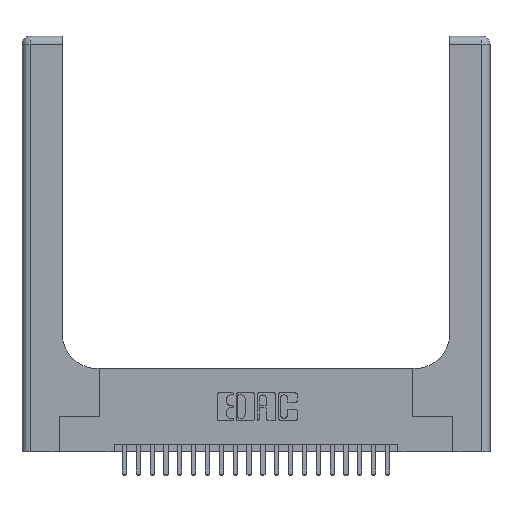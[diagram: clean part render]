
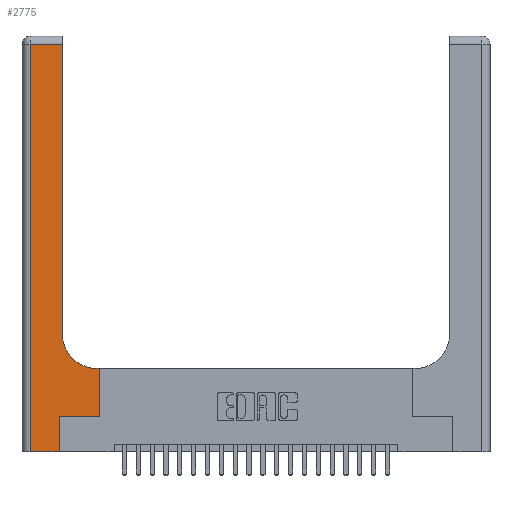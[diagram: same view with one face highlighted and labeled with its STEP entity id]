
A CAD part, top view. The second image highlights one B-rep face of the part: STEP entity #2775.
In plain terms, the highlighted planar face has unit normal (0, 0, 1).
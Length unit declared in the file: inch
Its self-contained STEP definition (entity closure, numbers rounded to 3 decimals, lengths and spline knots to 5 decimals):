
#641 = FACE_OUTER_BOUND ( 'NONE', #3121, .T. ) ;
#730 = VERTEX_POINT ( 'NONE', #21293 ) ;
#786 = ORIENTED_EDGE ( 'NONE', *, *, #1810, .T. ) ;
#1066 = CARTESIAN_POINT ( 'NONE',  ( 0., 3., 0.37 ) ) ;
#1249 = ORIENTED_EDGE ( 'NONE', *, *, #1352, .T. ) ;
#1352 = EDGE_CURVE ( 'NONE', #17365, #7725, #15824, .T. ) ;
#1807 = VECTOR ( 'NONE', #14139, 39.37008 ) ;
#1810 = EDGE_CURVE ( 'NONE', #20880, #12231, #6983, .T. ) ;
#1857 = CARTESIAN_POINT ( 'NONE',  ( 0.06, 0., 0.37 ) ) ;
#2157 = CARTESIAN_POINT ( 'NONE',  ( 0.06, 3., 0.37 ) ) ;
#2266 = VECTOR ( 'NONE', #17331, 39.37008 ) ;
#2618 = LINE ( 'NONE', #9656, #8392 ) ;
#2775 = ADVANCED_FACE ( 'NONE', ( #641 ), #12536, .F. ) ;
#3005 = DIRECTION ( 'NONE',  ( 0., 0., -1. ) ) ;
#3024 = VERTEX_POINT ( 'NONE', #22184 ) ;
#3121 = EDGE_LOOP ( 'NONE', ( #19429, #1249, #23349, #786, #3945, #17638, #7625, #6268, #14112 ) ) ;
#3131 = EDGE_CURVE ( 'NONE', #7725, #20880, #22711, .T. ) ;
#3136 = DIRECTION ( 'NONE',  ( -1., 0., 0. ) ) ;
#3695 = CARTESIAN_POINT ( 'NONE',  ( 0.269, 0., 0.37 ) ) ;
#3855 = EDGE_CURVE ( 'NONE', #11479, #17365, #17813, .T. ) ;
#3945 = ORIENTED_EDGE ( 'NONE', *, *, #23027, .T. ) ;
#4457 = DIRECTION ( 'NONE',  ( 0., 1., 0. ) ) ;
#5691 = CARTESIAN_POINT ( 'NONE',  ( 0., 2.94, 0.37 ) ) ;
#5713 = EDGE_CURVE ( 'NONE', #3024, #16464, #2618, .T. ) ;
#6214 = CIRCLE ( 'NONE', #7340, 0.25 ) ;
#6268 = ORIENTED_EDGE ( 'NONE', *, *, #5713, .T. ) ;
#6983 = LINE ( 'NONE', #18980, #1807 ) ;
#7340 = AXIS2_PLACEMENT_3D ( 'NONE', #9817, #22470, #11686 ) ;
#7625 = ORIENTED_EDGE ( 'NONE', *, *, #22004, .T. ) ;
#7725 = VERTEX_POINT ( 'NONE', #22381 ) ;
#7817 = CARTESIAN_POINT ( 'NONE',  ( 0.2915, 0.85, 0.37 ) ) ;
#8392 = VECTOR ( 'NONE', #22313, 39.37008 ) ;
#8693 = AXIS2_PLACEMENT_3D ( 'NONE', #1066, #3005, #16290 ) ;
#8915 = VECTOR ( 'NONE', #23266, 39.37008 ) ;
#9656 = CARTESIAN_POINT ( 'NONE',  ( 0.2915, 0.6, 0.37 ) ) ;
#9817 = CARTESIAN_POINT ( 'NONE',  ( 0.5415, 0.85, 0.37 ) ) ;
#10864 = VECTOR ( 'NONE', #3136, 39.37008 ) ;
#11479 = VERTEX_POINT ( 'NONE', #7817 ) ;
#11655 = CARTESIAN_POINT ( 'NONE',  ( 0.269, 0., 0.37 ) ) ;
#11686 = DIRECTION ( 'NONE',  ( 1., 0., 0. ) ) ;
#11877 = CARTESIAN_POINT ( 'NONE',  ( 0.269, 0.25, 0.37 ) ) ;
#12231 = VERTEX_POINT ( 'NONE', #11655 ) ;
#12536 = PLANE ( 'NONE',  #8693 ) ;
#12798 = LINE ( 'NONE', #3695, #17161 ) ;
#12887 = VECTOR ( 'NONE', #4457, 39.37008 ) ;
#13097 = CARTESIAN_POINT ( 'NONE',  ( 0.5415, 0.6, 0.37 ) ) ;
#13219 = DIRECTION ( 'NONE',  ( 0., 1., 0. ) ) ;
#13591 = DIRECTION ( 'NONE',  ( 0., -1., 0. ) ) ;
#14112 = ORIENTED_EDGE ( 'NONE', *, *, #23763, .T. ) ;
#14139 = DIRECTION ( 'NONE',  ( 1., 0., 0. ) ) ;
#15080 = EDGE_CURVE ( 'NONE', #23720, #730, #19283, .T. ) ;
#15487 = CARTESIAN_POINT ( 'NONE',  ( 0.5585, 0.25, 0.37 ) ) ;
#15824 = LINE ( 'NONE', #5691, #10864 ) ;
#15841 = CARTESIAN_POINT ( 'NONE',  ( 0.2915, 3., 0.37 ) ) ;
#16290 = DIRECTION ( 'NONE',  ( -1., 0., 0. ) ) ;
#16464 = VERTEX_POINT ( 'NONE', #13097 ) ;
#17161 = VECTOR ( 'NONE', #13219, 39.37008 ) ;
#17331 = DIRECTION ( 'NONE',  ( 0., 1., 0. ) ) ;
#17365 = VERTEX_POINT ( 'NONE', #18158 ) ;
#17387 = LINE ( 'NONE', #15487, #2266 ) ;
#17638 = ORIENTED_EDGE ( 'NONE', *, *, #15080, .T. ) ;
#17813 = LINE ( 'NONE', #15841, #12887 ) ;
#18125 = VECTOR ( 'NONE', #13591, 39.37008 ) ;
#18158 = CARTESIAN_POINT ( 'NONE',  ( 0.2915, 2.94, 0.37 ) ) ;
#18804 = CARTESIAN_POINT ( 'NONE',  ( 0.269, 0.25, 0.37 ) ) ;
#18980 = CARTESIAN_POINT ( 'NONE',  ( 0., 0., 0.37 ) ) ;
#19283 = LINE ( 'NONE', #18804, #8915 ) ;
#19429 = ORIENTED_EDGE ( 'NONE', *, *, #3855, .T. ) ;
#20880 = VERTEX_POINT ( 'NONE', #1857 ) ;
#21293 = CARTESIAN_POINT ( 'NONE',  ( 0.5585, 0.25, 0.37 ) ) ;
#22004 = EDGE_CURVE ( 'NONE', #730, #3024, #17387, .T. ) ;
#22184 = CARTESIAN_POINT ( 'NONE',  ( 0.5585, 0.6, 0.37 ) ) ;
#22313 = DIRECTION ( 'NONE',  ( -1., 0., 0. ) ) ;
#22381 = CARTESIAN_POINT ( 'NONE',  ( 0.06, 2.94, 0.37 ) ) ;
#22470 = DIRECTION ( 'NONE',  ( 0., 0., -1. ) ) ;
#22711 = LINE ( 'NONE', #2157, #18125 ) ;
#23027 = EDGE_CURVE ( 'NONE', #12231, #23720, #12798, .T. ) ;
#23266 = DIRECTION ( 'NONE',  ( 1., 0., 0. ) ) ;
#23349 = ORIENTED_EDGE ( 'NONE', *, *, #3131, .T. ) ;
#23720 = VERTEX_POINT ( 'NONE', #11877 ) ;
#23763 = EDGE_CURVE ( 'NONE', #16464, #11479, #6214, .T. ) ;
